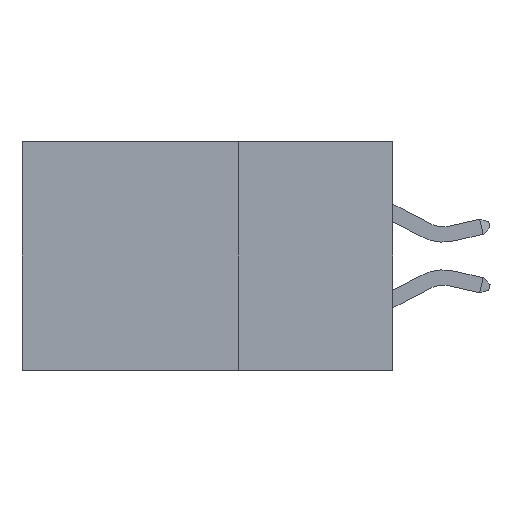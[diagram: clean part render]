
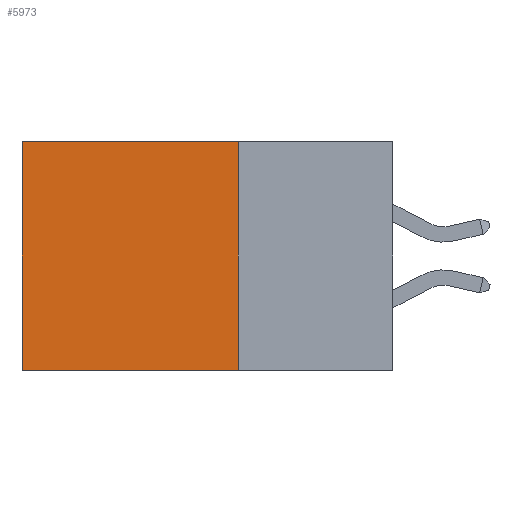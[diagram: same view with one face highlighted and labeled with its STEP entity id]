
A CAD part, left-side view. The second image highlights one B-rep face of the part: STEP entity #5973.
In plain terms, the highlighted planar face has unit normal (-1, 0, 0).
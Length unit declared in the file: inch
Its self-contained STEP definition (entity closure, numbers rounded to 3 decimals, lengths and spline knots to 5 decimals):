
#216 = DIRECTION ( 'NONE',  ( 1., 0., 0. ) ) ;
#461 = PLANE ( 'NONE',  #11464 ) ;
#1341 = VERTEX_POINT ( 'NONE', #3917 ) ;
#1426 = CARTESIAN_POINT ( 'NONE',  ( 0.2875, 0.6, 0. ) ) ;
#1757 = DIRECTION ( 'NONE',  ( 0., 1., 0. ) ) ;
#2071 = EDGE_CURVE ( 'NONE', #2155, #6514, #9204, .T. ) ;
#2155 = VERTEX_POINT ( 'NONE', #5321 ) ;
#2198 = DIRECTION ( 'NONE',  ( 0., 0., -1. ) ) ;
#2682 = ORIENTED_EDGE ( 'NONE', *, *, #6327, .T. ) ;
#3031 = CARTESIAN_POINT ( 'NONE',  ( 0.2875, 0.6, 0. ) ) ;
#3051 = CARTESIAN_POINT ( 'NONE',  ( 0.2875, 0.25, 0. ) ) ;
#3407 = EDGE_LOOP ( 'NONE', ( #2682, #11925, #11677, #10221 ) ) ;
#3602 = DIRECTION ( 'NONE',  ( 0., 0., -1. ) ) ;
#3617 = FACE_OUTER_BOUND ( 'NONE', #3407, .T. ) ;
#3917 = CARTESIAN_POINT ( 'NONE',  ( 0.2875, 0.25, 0. ) ) ;
#4303 = DIRECTION ( 'NONE',  ( 0., 0., -1. ) ) ;
#5321 = CARTESIAN_POINT ( 'NONE',  ( 0.2875, 0.25, -0.37 ) ) ;
#5785 = VECTOR ( 'NONE', #3602, 39.37008 ) ;
#5822 = VECTOR ( 'NONE', #1757, 39.37008 ) ;
#5973 = ADVANCED_FACE ( 'NONE', ( #3617 ), #461, .F. ) ;
#6327 = EDGE_CURVE ( 'NONE', #8093, #6514, #7417, .T. ) ;
#6374 = LINE ( 'NONE', #8290, #5785 ) ;
#6514 = VERTEX_POINT ( 'NONE', #11277 ) ;
#7146 = LINE ( 'NONE', #12116, #5822 ) ;
#7417 = LINE ( 'NONE', #1426, #9551 ) ;
#7732 = EDGE_CURVE ( 'NONE', #1341, #2155, #6374, .T. ) ;
#8093 = VERTEX_POINT ( 'NONE', #3031 ) ;
#8290 = CARTESIAN_POINT ( 'NONE',  ( 0.2875, 0.25, 0. ) ) ;
#8821 = DIRECTION ( 'NONE',  ( 0., 1., 0. ) ) ;
#9002 = EDGE_CURVE ( 'NONE', #1341, #8093, #7146, .T. ) ;
#9204 = LINE ( 'NONE', #9748, #11482 ) ;
#9551 = VECTOR ( 'NONE', #2198, 39.37008 ) ;
#9748 = CARTESIAN_POINT ( 'NONE',  ( 0.2875, 0.25, -0.37 ) ) ;
#10221 = ORIENTED_EDGE ( 'NONE', *, *, #9002, .T. ) ;
#11277 = CARTESIAN_POINT ( 'NONE',  ( 0.2875, 0.6, -0.37 ) ) ;
#11464 = AXIS2_PLACEMENT_3D ( 'NONE', #3051, #216, #4303 ) ;
#11482 = VECTOR ( 'NONE', #8821, 39.37008 ) ;
#11677 = ORIENTED_EDGE ( 'NONE', *, *, #7732, .F. ) ;
#11925 = ORIENTED_EDGE ( 'NONE', *, *, #2071, .F. ) ;
#12116 = CARTESIAN_POINT ( 'NONE',  ( 0.2875, 0.25, 0. ) ) ;
